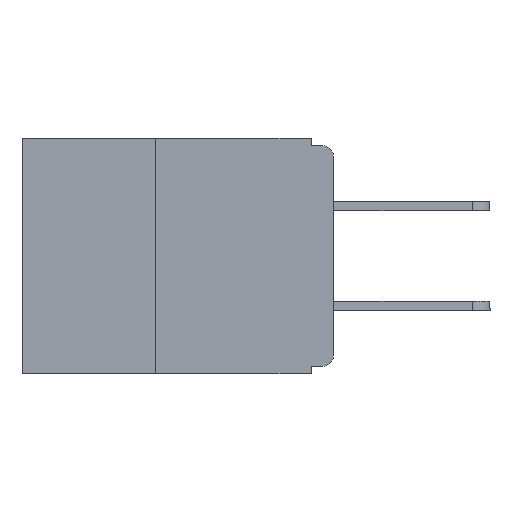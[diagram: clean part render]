
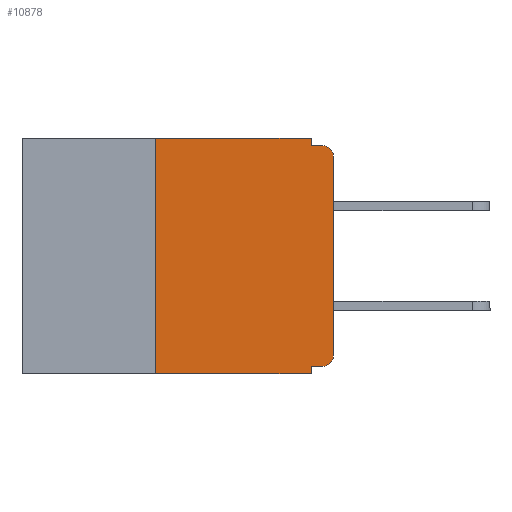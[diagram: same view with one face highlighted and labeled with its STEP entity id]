
A CAD part, left-side view. The second image highlights one B-rep face of the part: STEP entity #10878.
In plain terms, the highlighted planar face has unit normal (-1, 0, 0).
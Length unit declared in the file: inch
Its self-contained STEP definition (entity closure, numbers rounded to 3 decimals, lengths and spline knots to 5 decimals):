
#549 = DIRECTION ( 'NONE',  ( 0., 0., -1. ) ) ;
#589 = VERTEX_POINT ( 'NONE', #11465 ) ;
#771 = EDGE_CURVE ( 'NONE', #32697, #30663, #24172, .T. ) ;
#924 = CARTESIAN_POINT ( 'NONE',  ( 0., 0.25, 0. ) ) ;
#1152 = DIRECTION ( 'NONE',  ( 0., 0., 1. ) ) ;
#1838 = CARTESIAN_POINT ( 'NONE',  ( 0., 0.25, -0.33 ) ) ;
#2151 = FACE_OUTER_BOUND ( 'NONE', #28315, .T. ) ;
#2264 = CARTESIAN_POINT ( 'NONE',  ( 0., 0., 0. ) ) ;
#2421 = DIRECTION ( 'NONE',  ( 0., -1., 0. ) ) ;
#2461 = CARTESIAN_POINT ( 'NONE',  ( 0., 0.015, -0.01 ) ) ;
#2670 = ORIENTED_EDGE ( 'NONE', *, *, #28561, .F. ) ;
#3140 = CARTESIAN_POINT ( 'NONE',  ( 0., 0.437, 0. ) ) ;
#3218 = ORIENTED_EDGE ( 'NONE', *, *, #21132, .F. ) ;
#3639 = VECTOR ( 'NONE', #9194, 39.37008 ) ;
#4074 = LINE ( 'NONE', #29165, #30117 ) ;
#4811 = DIRECTION ( 'NONE',  ( 0., -1., 0. ) ) ;
#5028 = DIRECTION ( 'NONE',  ( 0., 0., 1. ) ) ;
#5329 = LINE ( 'NONE', #10459, #18505 ) ;
#5358 = DIRECTION ( 'NONE',  ( -1., 0., 0. ) ) ;
#5466 = LINE ( 'NONE', #31949, #18629 ) ;
#5701 = AXIS2_PLACEMENT_3D ( 'NONE', #33320, #30232, #30013 ) ;
#5856 = EDGE_CURVE ( 'NONE', #17169, #589, #17022, .T. ) ;
#5894 = ORIENTED_EDGE ( 'NONE', *, *, #5856, .T. ) ;
#6530 = CARTESIAN_POINT ( 'NONE',  ( 0., 0.031, -0.33 ) ) ;
#7355 = LINE ( 'NONE', #32788, #14348 ) ;
#8612 = DIRECTION ( 'NONE',  ( 0., 0., -1. ) ) ;
#8831 = EDGE_CURVE ( 'NONE', #32697, #25716, #5329, .T. ) ;
#9194 = DIRECTION ( 'NONE',  ( 0., 1., 0. ) ) ;
#9853 = EDGE_CURVE ( 'NONE', #31328, #11436, #7355, .T. ) ;
#10459 = CARTESIAN_POINT ( 'NONE',  ( 0., 0.437, -0.33 ) ) ;
#10609 = CARTESIAN_POINT ( 'NONE',  ( 0., 0.015, -0.32 ) ) ;
#10878 = ADVANCED_FACE ( 'NONE', ( #2151 ), #19001, .F. ) ;
#11030 = LINE ( 'NONE', #25610, #17157 ) ;
#11144 = ORIENTED_EDGE ( 'NONE', *, *, #13606, .F. ) ;
#11436 = VERTEX_POINT ( 'NONE', #23816 ) ;
#11460 = AXIS2_PLACEMENT_3D ( 'NONE', #21112, #5358, #23687 ) ;
#11465 = CARTESIAN_POINT ( 'NONE',  ( 0., 0., -0.305 ) ) ;
#12241 = AXIS2_PLACEMENT_3D ( 'NONE', #3140, #24175, #8612 ) ;
#12349 = CARTESIAN_POINT ( 'NONE',  ( 0., 0.031, -0.32 ) ) ;
#13606 = EDGE_CURVE ( 'NONE', #30663, #31328, #11030, .T. ) ;
#13773 = DIRECTION ( 'NONE',  ( 0., -1., 0. ) ) ;
#14348 = VECTOR ( 'NONE', #30331, 39.37008 ) ;
#16162 = CIRCLE ( 'NONE', #11460, 0.015 ) ;
#17022 = CIRCLE ( 'NONE', #5701, 0.015 ) ;
#17157 = VECTOR ( 'NONE', #4811, 39.37008 ) ;
#17169 = VERTEX_POINT ( 'NONE', #10609 ) ;
#17314 = VECTOR ( 'NONE', #1152, 39.37008 ) ;
#17598 = ORIENTED_EDGE ( 'NONE', *, *, #29102, .T. ) ;
#18144 = CARTESIAN_POINT ( 'NONE',  ( 0., 0., -0.025 ) ) ;
#18505 = VECTOR ( 'NONE', #2421, 39.37008 ) ;
#18506 = LINE ( 'NONE', #2264, #31258 ) ;
#18629 = VECTOR ( 'NONE', #549, 39.37008 ) ;
#19001 = PLANE ( 'NONE',  #12241 ) ;
#20945 = EDGE_CURVE ( 'NONE', #11436, #28832, #4074, .T. ) ;
#21112 = CARTESIAN_POINT ( 'NONE',  ( 0., 0.015, -0.025 ) ) ;
#21132 = EDGE_CURVE ( 'NONE', #17169, #25206, #25356, .T. ) ;
#22055 = VERTEX_POINT ( 'NONE', #18144 ) ;
#22847 = ORIENTED_EDGE ( 'NONE', *, *, #771, .F. ) ;
#22993 = ORIENTED_EDGE ( 'NONE', *, *, #8831, .T. ) ;
#23687 = DIRECTION ( 'NONE',  ( 0., 0., -1. ) ) ;
#23816 = CARTESIAN_POINT ( 'NONE',  ( 0., 0.031, -0.01 ) ) ;
#24172 = LINE ( 'NONE', #1838, #17314 ) ;
#24175 = DIRECTION ( 'NONE',  ( 1., 0., 0. ) ) ;
#24561 = CARTESIAN_POINT ( 'NONE',  ( 0., 0.25, -0.33 ) ) ;
#25172 = ORIENTED_EDGE ( 'NONE', *, *, #9853, .F. ) ;
#25206 = VERTEX_POINT ( 'NONE', #12349 ) ;
#25356 = LINE ( 'NONE', #29810, #3639 ) ;
#25610 = CARTESIAN_POINT ( 'NONE',  ( 0., 0.437, 0. ) ) ;
#25716 = VERTEX_POINT ( 'NONE', #6530 ) ;
#27830 = CARTESIAN_POINT ( 'NONE',  ( 0., 0.031, 0. ) ) ;
#28315 = EDGE_LOOP ( 'NONE', ( #32282, #17598, #33193, #25172, #11144, #22847, #22993, #2670, #3218, #5894 ) ) ;
#28561 = EDGE_CURVE ( 'NONE', #25206, #25716, #5466, .T. ) ;
#28832 = VERTEX_POINT ( 'NONE', #2461 ) ;
#29102 = EDGE_CURVE ( 'NONE', #22055, #28832, #16162, .T. ) ;
#29165 = CARTESIAN_POINT ( 'NONE',  ( 0., 0., -0.01 ) ) ;
#29810 = CARTESIAN_POINT ( 'NONE',  ( 0., 0., -0.32 ) ) ;
#30013 = DIRECTION ( 'NONE',  ( 0., 0., -1. ) ) ;
#30117 = VECTOR ( 'NONE', #13773, 39.37008 ) ;
#30232 = DIRECTION ( 'NONE',  ( -1., 0., 0. ) ) ;
#30315 = EDGE_CURVE ( 'NONE', #589, #22055, #18506, .T. ) ;
#30331 = DIRECTION ( 'NONE',  ( 0., 0., -1. ) ) ;
#30663 = VERTEX_POINT ( 'NONE', #924 ) ;
#31258 = VECTOR ( 'NONE', #5028, 39.37008 ) ;
#31328 = VERTEX_POINT ( 'NONE', #27830 ) ;
#31949 = CARTESIAN_POINT ( 'NONE',  ( 0., 0.031, -0.33 ) ) ;
#32282 = ORIENTED_EDGE ( 'NONE', *, *, #30315, .T. ) ;
#32697 = VERTEX_POINT ( 'NONE', #24561 ) ;
#32788 = CARTESIAN_POINT ( 'NONE',  ( 0., 0.031, 0. ) ) ;
#33193 = ORIENTED_EDGE ( 'NONE', *, *, #20945, .F. ) ;
#33320 = CARTESIAN_POINT ( 'NONE',  ( 0., 0.015, -0.305 ) ) ;
